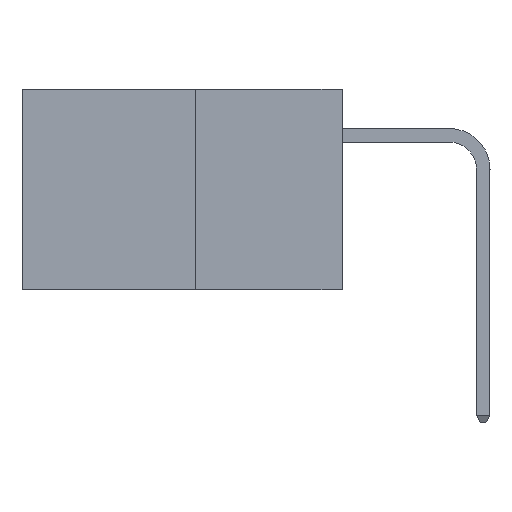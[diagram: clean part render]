
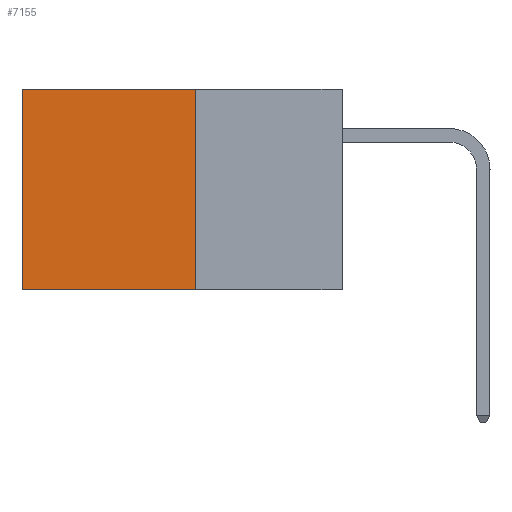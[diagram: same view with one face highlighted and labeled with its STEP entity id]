
A CAD part, left-side view. The second image highlights one B-rep face of the part: STEP entity #7155.
In plain terms, the highlighted planar face has unit normal (-1, 0, 0).
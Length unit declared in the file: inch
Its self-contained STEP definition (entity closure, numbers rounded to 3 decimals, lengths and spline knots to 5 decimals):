
#1573 = FACE_OUTER_BOUND ( 'NONE', #17651, .T. ) ;
#2130 = VECTOR ( 'NONE', #7039, 39.37008 ) ;
#2552 = VECTOR ( 'NONE', #18659, 39.37008 ) ;
#2890 = DIRECTION ( 'NONE',  ( 0., 1., 0. ) ) ;
#3084 = PLANE ( 'NONE',  #16554 ) ;
#3633 = LINE ( 'NONE', #10962, #19612 ) ;
#5644 = VERTEX_POINT ( 'NONE', #8146 ) ;
#6751 = VECTOR ( 'NONE', #13654, 39.37008 ) ;
#6903 = EDGE_CURVE ( 'NONE', #12687, #18012, #15261, .T. ) ;
#7039 = DIRECTION ( 'NONE',  ( 0., 1., 0. ) ) ;
#7155 = ADVANCED_FACE ( 'NONE', ( #1573 ), #3084, .F. ) ;
#7213 = ORIENTED_EDGE ( 'NONE', *, *, #18324, .T. ) ;
#7422 = VERTEX_POINT ( 'NONE', #19832 ) ;
#8146 = CARTESIAN_POINT ( 'NONE',  ( 0.277, 0.27, -0.37 ) ) ;
#8552 = ORIENTED_EDGE ( 'NONE', *, *, #15440, .F. ) ;
#9116 = CARTESIAN_POINT ( 'NONE',  ( 0.277, 0.27, -0.37 ) ) ;
#9767 = LINE ( 'NONE', #16594, #2130 ) ;
#10962 = CARTESIAN_POINT ( 'NONE',  ( 0.277, 0.27, -0.37 ) ) ;
#11043 = CARTESIAN_POINT ( 'NONE',  ( 0.277, 0.59, -0.37 ) ) ;
#12687 = VERTEX_POINT ( 'NONE', #15671 ) ;
#13654 = DIRECTION ( 'NONE',  ( 0., 0., -1. ) ) ;
#14598 = ORIENTED_EDGE ( 'NONE', *, *, #6903, .T. ) ;
#15261 = LINE ( 'NONE', #17735, #6751 ) ;
#15433 = LINE ( 'NONE', #9116, #2552 ) ;
#15440 = EDGE_CURVE ( 'NONE', #7422, #5644, #15433, .T. ) ;
#15671 = CARTESIAN_POINT ( 'NONE',  ( 0.277, 0.59, 0. ) ) ;
#16364 = DIRECTION ( 'NONE',  ( 0., 0., -1. ) ) ;
#16554 = AXIS2_PLACEMENT_3D ( 'NONE', #19404, #19306, #16364 ) ;
#16594 = CARTESIAN_POINT ( 'NONE',  ( 0.277, 0.27, 0. ) ) ;
#17486 = ORIENTED_EDGE ( 'NONE', *, *, #20161, .F. ) ;
#17651 = EDGE_LOOP ( 'NONE', ( #14598, #17486, #8552, #7213 ) ) ;
#17735 = CARTESIAN_POINT ( 'NONE',  ( 0.277, 0.59, -0.37 ) ) ;
#18012 = VERTEX_POINT ( 'NONE', #11043 ) ;
#18324 = EDGE_CURVE ( 'NONE', #7422, #12687, #9767, .T. ) ;
#18659 = DIRECTION ( 'NONE',  ( 0., 0., -1. ) ) ;
#19306 = DIRECTION ( 'NONE',  ( 1., 0., 0. ) ) ;
#19404 = CARTESIAN_POINT ( 'NONE',  ( 0.277, 0.27, -0.37 ) ) ;
#19612 = VECTOR ( 'NONE', #2890, 39.37008 ) ;
#19832 = CARTESIAN_POINT ( 'NONE',  ( 0.277, 0.27, 0. ) ) ;
#20161 = EDGE_CURVE ( 'NONE', #5644, #18012, #3633, .T. ) ;
